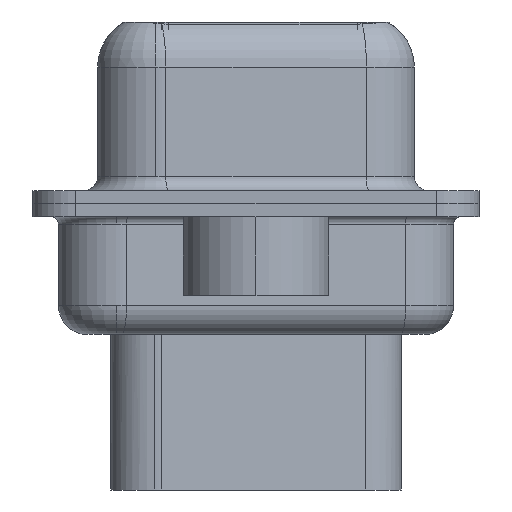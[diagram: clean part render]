
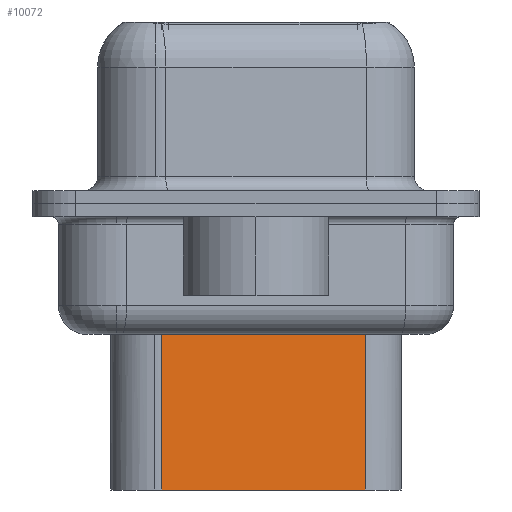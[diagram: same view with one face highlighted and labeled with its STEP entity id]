
A CAD part, left-side view. The second image highlights one B-rep face of the part: STEP entity #10072.
In plain terms, the highlighted planar face has unit normal (-0.985, -0.174, 0).
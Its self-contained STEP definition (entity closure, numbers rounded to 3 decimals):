
#4459 = EDGE_CURVE ( 'NONE', #32399, #20950, #19129, .T. ) ;
#5721 = CARTESIAN_POINT ( 'NONE',  ( 4.624, 3.24, -3.1 ) ) ;
#5732 = CARTESIAN_POINT ( 'NONE',  ( 4.624, 3.24, -9.85 ) ) ;
#6005 = LINE ( 'NONE', #17655, #25073 ) ;
#8125 = EDGE_CURVE ( 'NONE', #32399, #10058, #36077, .T. ) ;
#8781 = DIRECTION ( 'NONE',  ( -0.985, -0.174, 0. ) ) ;
#9944 = VECTOR ( 'NONE', #27047, 1000. ) ;
#10058 = VERTEX_POINT ( 'NONE', #14892 ) ;
#10072 = ADVANCED_FACE ( 'NONE', ( #14699 ), #26328, .T. ) ;
#10583 = EDGE_CURVE ( 'NONE', #10058, #19126, #24573, .T. ) ;
#11728 = EDGE_LOOP ( 'NONE', ( #30123, #37541, #37624, #31637 ) ) ;
#14699 = FACE_OUTER_BOUND ( 'NONE', #11728, .T. ) ;
#14892 = CARTESIAN_POINT ( 'NONE',  ( 4.624, 3.24, -3.975 ) ) ;
#15407 = CARTESIAN_POINT ( 'NONE',  ( 4.624, 3.24, -3.1 ) ) ;
#17655 = CARTESIAN_POINT ( 'NONE',  ( 4.624, 3.24, -9.85 ) ) ;
#19116 = AXIS2_PLACEMENT_3D ( 'NONE', #5721, #8781, #28990 ) ;
#19126 = VERTEX_POINT ( 'NONE', #5732 ) ;
#19129 = LINE ( 'NONE', #25038, #25825 ) ;
#19676 = DIRECTION ( 'NONE',  ( 0., 0., -1. ) ) ;
#20950 = VERTEX_POINT ( 'NONE', #31160 ) ;
#24573 = LINE ( 'NONE', #15407, #9944 ) ;
#25038 = CARTESIAN_POINT ( 'NONE',  ( 5.858, -3.76, -3.1 ) ) ;
#25073 = VECTOR ( 'NONE', #29276, 1000. ) ;
#25825 = VECTOR ( 'NONE', #19676, 1000. ) ;
#26328 = PLANE ( 'NONE',  #19116 ) ;
#27047 = DIRECTION ( 'NONE',  ( 0., 0., -1. ) ) ;
#28990 = DIRECTION ( 'NONE',  ( 0.174, -0.985, 0. ) ) ;
#29277 = EDGE_CURVE ( 'NONE', #20950, #19126, #6005, .T. ) ;
#29276 = DIRECTION ( 'NONE',  ( -0.174, 0.985, 0. ) ) ;
#29770 = VECTOR ( 'NONE', #33220, 1000. ) ;
#30123 = ORIENTED_EDGE ( 'NONE', *, *, #4459, .F. ) ;
#31160 = CARTESIAN_POINT ( 'NONE',  ( 5.858, -3.76, -9.85 ) ) ;
#31637 = ORIENTED_EDGE ( 'NONE', *, *, #29277, .F. ) ;
#32399 = VERTEX_POINT ( 'NONE', #33752 ) ;
#33027 = CARTESIAN_POINT ( 'NONE',  ( 4.453, 4.209, -3.975 ) ) ;
#33220 = DIRECTION ( 'NONE',  ( -0.174, 0.985, 0. ) ) ;
#33752 = CARTESIAN_POINT ( 'NONE',  ( 5.858, -3.76, -3.975 ) ) ;
#36077 = LINE ( 'NONE', #33027, #29770 ) ;
#37541 = ORIENTED_EDGE ( 'NONE', *, *, #8125, .T. ) ;
#37624 = ORIENTED_EDGE ( 'NONE', *, *, #10583, .T. ) ;
